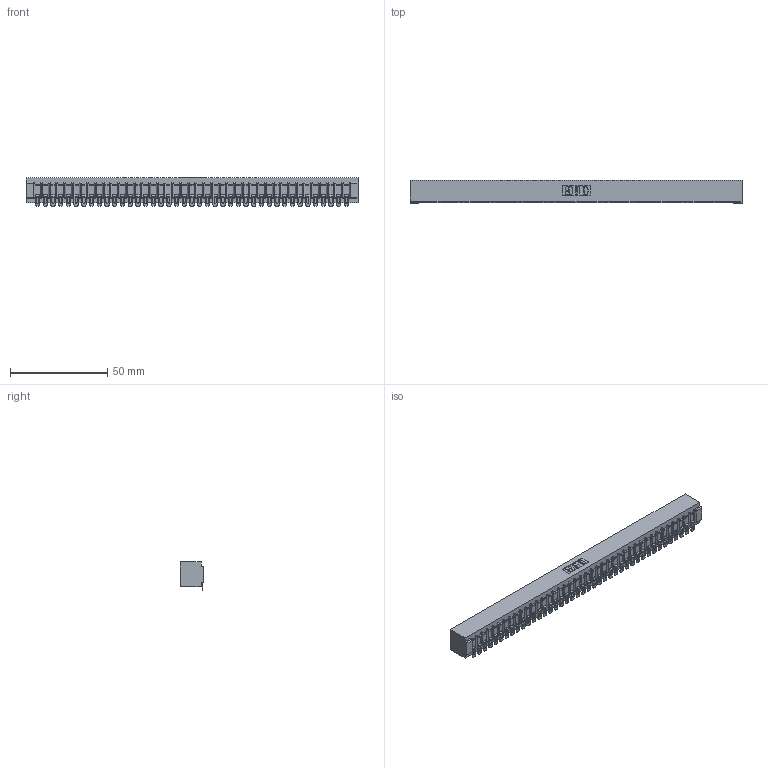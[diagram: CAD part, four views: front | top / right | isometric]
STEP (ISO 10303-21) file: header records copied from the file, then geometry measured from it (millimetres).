
FILE_DESCRIPTION (( 'STEP AP203' ), '1' );
FILE_NAME ('307-041-454-101.STEP', '2020-09-29T16:11:47', ( '' ), ( '' ), 'SwSTEP 2.0', 'SolidWorks 2020', '' );
FILE_SCHEMA (( 'CONFIG_CONTROL_DESIGN' ));
Length unit declared in the file: inch
Products named in the file (3): 307-290-002_554; 307-041-454-101; 307 Part_No Mounting Lugs
Assembly tree (42 placements, depth 2):
  307-041-454-101
    307 Part_No Mounting Lugs
    307-290-002_554  x41
Bounding box: 170.33 x 12.01 x 14.52 mm (x, y, z)
Volume: 18792.8 mm3; surface area: 24114.8 mm2
Topology: 42 solids, 42 shells, 3473 faces, 10672 edges, 7000 vertices
Faces by surface type: plane 1952, cylinder 1437, sphere 84
Entity records: 35959 total; most frequent: CARTESIAN_POINT 6066, ORIENTED_EDGE 6056, DIRECTION 5898, EDGE_CURVE 3028, VECTOR 2314, LINE 2314, VERTEX_POINT 1960, AXIS2_PLACEMENT_3D 1792
